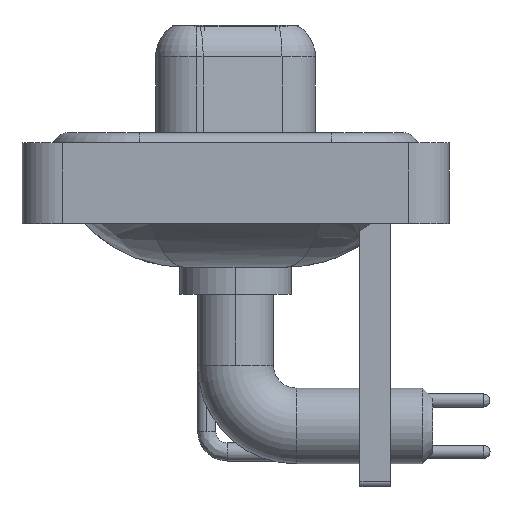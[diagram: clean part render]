
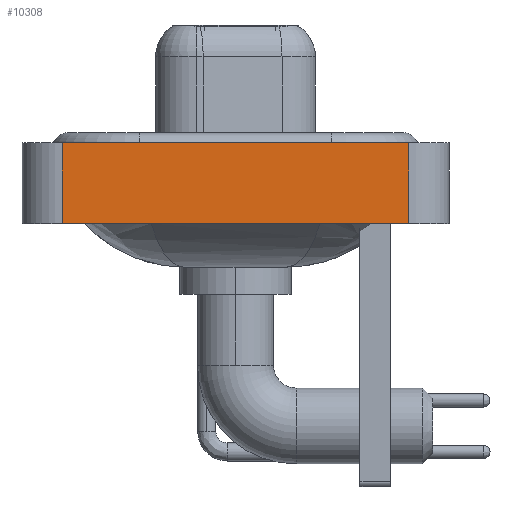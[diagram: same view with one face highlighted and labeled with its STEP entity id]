
A CAD part, left-side view. The second image highlights one B-rep face of the part: STEP entity #10308.
In plain terms, the highlighted planar face has unit normal (-1, 0, 0).
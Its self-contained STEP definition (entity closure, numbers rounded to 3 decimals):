
#581 = LINE ( 'NONE', #15390, #6817 ) ;
#1049 = CARTESIAN_POINT ( 'NONE',  ( -7.35, -8.55, -3.6 ) ) ;
#1131 = ORIENTED_EDGE ( 'NONE', *, *, #23602, .T. ) ;
#1804 = LINE ( 'NONE', #7294, #11858 ) ;
#2732 = ORIENTED_EDGE ( 'NONE', *, *, #15598, .T. ) ;
#2804 = AXIS2_PLACEMENT_3D ( 'NONE', #6899, #17855, #3535 ) ;
#2978 = ORIENTED_EDGE ( 'NONE', *, *, #16614, .F. ) ;
#3061 = VERTEX_POINT ( 'NONE', #6225 ) ;
#3535 = DIRECTION ( 'NONE',  ( 0., 0., 1. ) ) ;
#4062 = CARTESIAN_POINT ( 'NONE',  ( -7.35, -8.55, 0.4 ) ) ;
#5155 = DIRECTION ( 'NONE',  ( 0., -1., 0. ) ) ;
#5358 = VECTOR ( 'NONE', #15722, 1000. ) ;
#6225 = CARTESIAN_POINT ( 'NONE',  ( -7.35, 8.55, 0.4 ) ) ;
#6817 = VECTOR ( 'NONE', #15637, 1000. ) ;
#6899 = CARTESIAN_POINT ( 'NONE',  ( -7.35, -8.55, -3.6 ) ) ;
#7294 = CARTESIAN_POINT ( 'NONE',  ( -7.35, 8.55, -3.6 ) ) ;
#7421 = VERTEX_POINT ( 'NONE', #21899 ) ;
#9441 = EDGE_CURVE ( 'NONE', #7421, #3061, #1804, .T. ) ;
#10308 = ADVANCED_FACE ( 'NONE', ( #21788 ), #16203, .T. ) ;
#11858 = VECTOR ( 'NONE', #14568, 1000. ) ;
#12836 = VERTEX_POINT ( 'NONE', #14970 ) ;
#14094 = ORIENTED_EDGE ( 'NONE', *, *, #9441, .F. ) ;
#14228 = LINE ( 'NONE', #23293, #22580 ) ;
#14568 = DIRECTION ( 'NONE',  ( 0., 0., 1. ) ) ;
#14743 = VERTEX_POINT ( 'NONE', #4062 ) ;
#14970 = CARTESIAN_POINT ( 'NONE',  ( -7.35, -8.55, -3.6 ) ) ;
#15390 = CARTESIAN_POINT ( 'NONE',  ( -7.35, -8.55, -3.6 ) ) ;
#15598 = EDGE_CURVE ( 'NONE', #12836, #14743, #15840, .T. ) ;
#15637 = DIRECTION ( 'NONE',  ( 0., -1., 0. ) ) ;
#15722 = DIRECTION ( 'NONE',  ( 0., 0., 1. ) ) ;
#15840 = LINE ( 'NONE', #1049, #5358 ) ;
#16203 = PLANE ( 'NONE',  #2804 ) ;
#16614 = EDGE_CURVE ( 'NONE', #3061, #14743, #14228, .T. ) ;
#17133 = EDGE_LOOP ( 'NONE', ( #2732, #2978, #14094, #1131 ) ) ;
#17855 = DIRECTION ( 'NONE',  ( -1., 0., 0. ) ) ;
#21788 = FACE_OUTER_BOUND ( 'NONE', #17133, .T. ) ;
#21899 = CARTESIAN_POINT ( 'NONE',  ( -7.35, 8.55, -3.6 ) ) ;
#22580 = VECTOR ( 'NONE', #5155, 1000. ) ;
#23293 = CARTESIAN_POINT ( 'NONE',  ( -7.35, -8.55, 0.4 ) ) ;
#23602 = EDGE_CURVE ( 'NONE', #7421, #12836, #581, .T. ) ;
